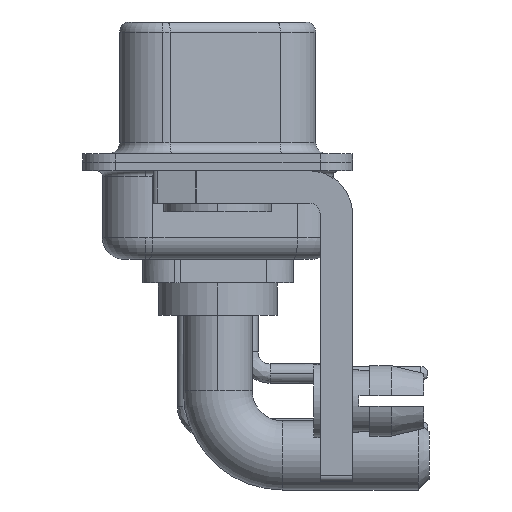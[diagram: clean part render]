
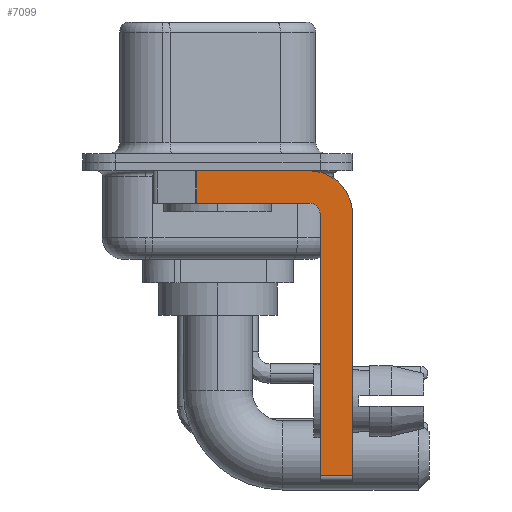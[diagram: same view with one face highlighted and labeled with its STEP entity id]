
A CAD part, left-side view. The second image highlights one B-rep face of the part: STEP entity #7099.
In plain terms, the highlighted planar face has unit normal (-1, 0, 0).
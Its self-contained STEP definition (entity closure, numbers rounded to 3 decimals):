
#234 = EDGE_CURVE ( 'NONE', #15248, #17216, #11147, .T. ) ;
#342 = CARTESIAN_POINT ( 'NONE',  ( -2.9, -4.25, -2.4 ) ) ;
#638 = CARTESIAN_POINT ( 'NONE',  ( -2.9, -4.25, -2.4 ) ) ;
#750 = LINE ( 'NONE', #4280, #4844 ) ;
#816 = DIRECTION ( 'NONE',  ( 0., -1., 0. ) ) ;
#1134 = DIRECTION ( 'NONE',  ( -1., 0., 0. ) ) ;
#1164 = EDGE_CURVE ( 'NONE', #4304, #15075, #750, .T. ) ;
#1709 = CARTESIAN_POINT ( 'NONE',  ( -2.9, 0.978, -0.4 ) ) ;
#1991 = ORIENTED_EDGE ( 'NONE', *, *, #21193, .F. ) ;
#2410 = VECTOR ( 'NONE', #19311, 1000. ) ;
#3204 = CIRCLE ( 'NONE', #10015, 0.5 ) ;
#3312 = DIRECTION ( 'NONE',  ( 1., 0., 0. ) ) ;
#3567 = CARTESIAN_POINT ( 'NONE',  ( -2.9, -4.75, -14.55 ) ) ;
#4223 = CARTESIAN_POINT ( 'NONE',  ( -2.9, -4.25, -14.55 ) ) ;
#4238 = FACE_OUTER_BOUND ( 'NONE', #6281, .T. ) ;
#4280 = CARTESIAN_POINT ( 'NONE',  ( -2.9, -4.75, -14.8 ) ) ;
#4304 = VERTEX_POINT ( 'NONE', #3567 ) ;
#4360 = CARTESIAN_POINT ( 'NONE',  ( -2.9, -4.25, -1.9 ) ) ;
#4844 = VECTOR ( 'NONE', #17835, 1000. ) ;
#4975 = CARTESIAN_POINT ( 'NONE',  ( -2.9, -4.75, -2.4 ) ) ;
#6039 = CARTESIAN_POINT ( 'NONE',  ( -2.9, 3., -0.4 ) ) ;
#6281 = EDGE_LOOP ( 'NONE', ( #12941, #8506, #16749, #17541, #14935, #6372, #1991, #21971 ) ) ;
#6372 = ORIENTED_EDGE ( 'NONE', *, *, #14128, .T. ) ;
#6616 = CARTESIAN_POINT ( 'NONE',  ( -2.9, -4.25, -2.4 ) ) ;
#7099 = ADVANCED_FACE ( 'NONE', ( #4238 ), #14735, .F. ) ;
#7642 = CARTESIAN_POINT ( 'NONE',  ( -2.9, -6.25, -2.4 ) ) ;
#8506 = ORIENTED_EDGE ( 'NONE', *, *, #234, .T. ) ;
#8548 = LINE ( 'NONE', #17072, #19118 ) ;
#8600 = VERTEX_POINT ( 'NONE', #22996 ) ;
#8724 = AXIS2_PLACEMENT_3D ( 'NONE', #6616, #3312, #14271 ) ;
#8788 = DIRECTION ( 'NONE',  ( 0., 0., 1. ) ) ;
#8912 = DIRECTION ( 'NONE',  ( 0., 1., 0. ) ) ;
#10015 = AXIS2_PLACEMENT_3D ( 'NONE', #638, #1134, #8788 ) ;
#10389 = AXIS2_PLACEMENT_3D ( 'NONE', #342, #15536, #15900 ) ;
#10529 = LINE ( 'NONE', #6039, #18793 ) ;
#11147 = LINE ( 'NONE', #18935, #2410 ) ;
#12466 = CARTESIAN_POINT ( 'NONE',  ( -2.9, 0.978, -1.9 ) ) ;
#12941 = ORIENTED_EDGE ( 'NONE', *, *, #17583, .F. ) ;
#13709 = DIRECTION ( 'NONE',  ( 0., -1., 0. ) ) ;
#14128 = EDGE_CURVE ( 'NONE', #4304, #15608, #16139, .T. ) ;
#14271 = DIRECTION ( 'NONE',  ( 0., 0., -1. ) ) ;
#14501 = CARTESIAN_POINT ( 'NONE',  ( -2.9, -6.25, -14.55 ) ) ;
#14735 = PLANE ( 'NONE',  #8724 ) ;
#14935 = ORIENTED_EDGE ( 'NONE', *, *, #1164, .F. ) ;
#15075 = VERTEX_POINT ( 'NONE', #4975 ) ;
#15248 = VERTEX_POINT ( 'NONE', #1709 ) ;
#15256 = CIRCLE ( 'NONE', #10389, 2. ) ;
#15536 = DIRECTION ( 'NONE',  ( 1., 0., 0. ) ) ;
#15608 = VERTEX_POINT ( 'NONE', #14501 ) ;
#15900 = DIRECTION ( 'NONE',  ( 0., 0., -1. ) ) ;
#15908 = EDGE_CURVE ( 'NONE', #23824, #17216, #8548, .T. ) ;
#16139 = LINE ( 'NONE', #4223, #22663 ) ;
#16749 = ORIENTED_EDGE ( 'NONE', *, *, #15908, .F. ) ;
#17072 = CARTESIAN_POINT ( 'NONE',  ( -2.9, -4.25, -1.9 ) ) ;
#17216 = VERTEX_POINT ( 'NONE', #12466 ) ;
#17541 = ORIENTED_EDGE ( 'NONE', *, *, #20851, .F. ) ;
#17583 = EDGE_CURVE ( 'NONE', #15248, #8600, #10529, .T. ) ;
#17835 = DIRECTION ( 'NONE',  ( 0., 0., 1. ) ) ;
#18793 = VECTOR ( 'NONE', #13709, 1000. ) ;
#18935 = CARTESIAN_POINT ( 'NONE',  ( -2.9, 0.978, -1.9 ) ) ;
#19118 = VECTOR ( 'NONE', #8912, 1000. ) ;
#19311 = DIRECTION ( 'NONE',  ( 0., 0., -1. ) ) ;
#19445 = DIRECTION ( 'NONE',  ( 0., 0., -1. ) ) ;
#20851 = EDGE_CURVE ( 'NONE', #15075, #23824, #3204, .T. ) ;
#21193 = EDGE_CURVE ( 'NONE', #24330, #15608, #21469, .T. ) ;
#21469 = LINE ( 'NONE', #7642, #22478 ) ;
#21971 = ORIENTED_EDGE ( 'NONE', *, *, #23733, .F. ) ;
#22478 = VECTOR ( 'NONE', #19445, 1000. ) ;
#22663 = VECTOR ( 'NONE', #816, 1000. ) ;
#22996 = CARTESIAN_POINT ( 'NONE',  ( -2.9, -4.25, -0.4 ) ) ;
#23733 = EDGE_CURVE ( 'NONE', #8600, #24330, #15256, .T. ) ;
#23824 = VERTEX_POINT ( 'NONE', #4360 ) ;
#24018 = CARTESIAN_POINT ( 'NONE',  ( -2.9, -6.25, -2.4 ) ) ;
#24330 = VERTEX_POINT ( 'NONE', #24018 ) ;
